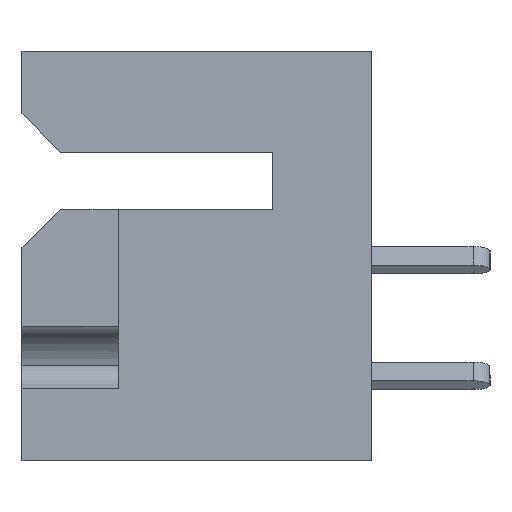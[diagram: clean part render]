
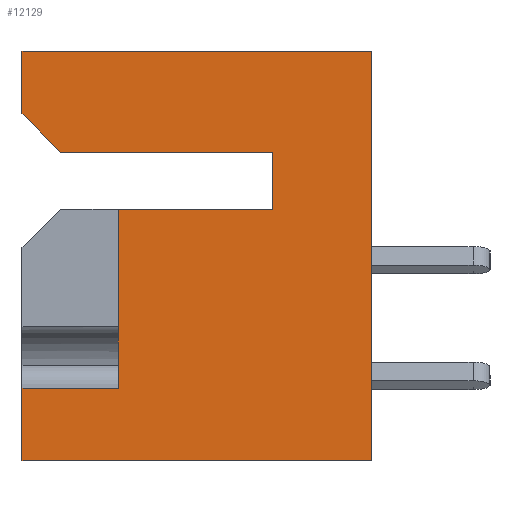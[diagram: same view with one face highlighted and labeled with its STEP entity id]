
A CAD part, left-side view. The second image highlights one B-rep face of the part: STEP entity #12129.
In plain terms, the highlighted planar face has unit normal (-1, 0, 0).
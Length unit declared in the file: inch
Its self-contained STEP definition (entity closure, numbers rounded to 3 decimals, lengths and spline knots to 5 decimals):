
#203 = ORIENTED_EDGE ( 'NONE', *, *, #2435, .F. ) ;
#369 = CARTESIAN_POINT ( 'NONE',  ( 0., 0.328, -0.437 ) ) ;
#496 = DIRECTION ( 'NONE',  ( 0., 1., 0. ) ) ;
#605 = LINE ( 'NONE', #17112, #13194 ) ;
#648 = LINE ( 'NONE', #10663, #18182 ) ;
#671 = DIRECTION ( 'NONE',  ( 0., 1., 0. ) ) ;
#907 = EDGE_CURVE ( 'NONE', #3482, #4054, #5371, .T. ) ;
#1064 = VECTOR ( 'NONE', #8066, 39.37008 ) ;
#1455 = CARTESIAN_POINT ( 'NONE',  ( 0., 0.128, -0.131 ) ) ;
#1504 = CARTESIAN_POINT ( 'NONE',  ( 0., 0.453, -0.081 ) ) ;
#1509 = VERTEX_POINT ( 'NONE', #19637 ) ;
#1584 = VERTEX_POINT ( 'NONE', #2932 ) ;
#1660 = LINE ( 'NONE', #2164, #2198 ) ;
#1769 = CARTESIAN_POINT ( 'NONE',  ( 0., 0.453, 0. ) ) ;
#1850 = DIRECTION ( 'NONE',  ( 0., -0.707, -0.707 ) ) ;
#1857 = LINE ( 'NONE', #14590, #1064 ) ;
#2164 = CARTESIAN_POINT ( 'NONE',  ( 0., 0.328, -0.437 ) ) ;
#2198 = VECTOR ( 'NONE', #496, 39.37008 ) ;
#2222 = EDGE_CURVE ( 'NONE', #15832, #9952, #6212, .T. ) ;
#2435 = EDGE_CURVE ( 'NONE', #15832, #11811, #10362, .T. ) ;
#2499 = DIRECTION ( 'NONE',  ( 0., 0., -1. ) ) ;
#2746 = ORIENTED_EDGE ( 'NONE', *, *, #13058, .F. ) ;
#2792 = VERTEX_POINT ( 'NONE', #369 ) ;
#2932 = CARTESIAN_POINT ( 'NONE',  ( 0., 0., 0. ) ) ;
#3037 = DIRECTION ( 'NONE',  ( 0., 1., 0. ) ) ;
#3432 = VECTOR ( 'NONE', #13560, 39.37008 ) ;
#3482 = VERTEX_POINT ( 'NONE', #6215 ) ;
#3641 = EDGE_CURVE ( 'NONE', #2792, #1509, #1857, .T. ) ;
#3700 = EDGE_CURVE ( 'NONE', #17153, #14867, #10065, .T. ) ;
#4054 = VERTEX_POINT ( 'NONE', #17410 ) ;
#4182 = CARTESIAN_POINT ( 'NONE',  ( 0., 0.453, 0. ) ) ;
#4705 = CARTESIAN_POINT ( 'NONE',  ( 0., 0.453, -0.531 ) ) ;
#5371 = LINE ( 'NONE', #6681, #6901 ) ;
#5588 = ORIENTED_EDGE ( 'NONE', *, *, #3641, .F. ) ;
#5972 = VECTOR ( 'NONE', #19059, 39.37008 ) ;
#6212 = LINE ( 'NONE', #16836, #19392 ) ;
#6215 = CARTESIAN_POINT ( 'NONE',  ( 0., 0.128, -0.205 ) ) ;
#6281 = LINE ( 'NONE', #21240, #12495 ) ;
#6378 = CARTESIAN_POINT ( 'NONE',  ( 0., 0.403, -0.131 ) ) ;
#6535 = DIRECTION ( 'NONE',  ( 0., 0., 1. ) ) ;
#6681 = CARTESIAN_POINT ( 'NONE',  ( 0., 0.128, -0.131 ) ) ;
#6891 = EDGE_CURVE ( 'NONE', #14867, #1584, #648, .T. ) ;
#6901 = VECTOR ( 'NONE', #6535, 39.37008 ) ;
#7118 = CARTESIAN_POINT ( 'NONE',  ( 0., 0., -0.531 ) ) ;
#7164 = LINE ( 'NONE', #1455, #14645 ) ;
#7287 = ORIENTED_EDGE ( 'NONE', *, *, #3700, .T. ) ;
#7370 = EDGE_CURVE ( 'NONE', #2792, #17673, #1660, .T. ) ;
#8011 = EDGE_CURVE ( 'NONE', #17153, #17673, #12193, .T. ) ;
#8066 = DIRECTION ( 'NONE',  ( 0., 0., 1. ) ) ;
#8409 = CARTESIAN_POINT ( 'NONE',  ( 0., 0.453, 0. ) ) ;
#8447 = CARTESIAN_POINT ( 'NONE',  ( 0., 0.453, -0.531 ) ) ;
#9952 = VERTEX_POINT ( 'NONE', #6378 ) ;
#10065 = LINE ( 'NONE', #4705, #13427 ) ;
#10362 = LINE ( 'NONE', #4182, #5972 ) ;
#10663 = CARTESIAN_POINT ( 'NONE',  ( 0., 0., 0. ) ) ;
#10883 = CARTESIAN_POINT ( 'NONE',  ( 0., 0.453, 0. ) ) ;
#11220 = EDGE_CURVE ( 'NONE', #4054, #9952, #7164, .T. ) ;
#11272 = EDGE_LOOP ( 'NONE', ( #16988, #19853, #7287, #20043, #2746, #203, #15900, #20462, #14332, #11787, #5588 ) ) ;
#11350 = DIRECTION ( 'NONE',  ( 0., -1., 0. ) ) ;
#11787 = ORIENTED_EDGE ( 'NONE', *, *, #14834, .T. ) ;
#11811 = VERTEX_POINT ( 'NONE', #1769 ) ;
#12091 = DIRECTION ( 'NONE',  ( 0., 0., 1. ) ) ;
#12129 = ADVANCED_FACE ( 'NONE', ( #17731 ), #20214, .F. ) ;
#12193 = LINE ( 'NONE', #8409, #3432 ) ;
#12495 = VECTOR ( 'NONE', #11350, 39.37008 ) ;
#12849 = CARTESIAN_POINT ( 'NONE',  ( 0., 0.453, -0.437 ) ) ;
#13058 = EDGE_CURVE ( 'NONE', #11811, #1584, #6281, .T. ) ;
#13194 = VECTOR ( 'NONE', #671, 39.37008 ) ;
#13360 = AXIS2_PLACEMENT_3D ( 'NONE', #10883, #19062, #2499 ) ;
#13427 = VECTOR ( 'NONE', #16270, 39.37008 ) ;
#13560 = DIRECTION ( 'NONE',  ( 0., 0., 1. ) ) ;
#14332 = ORIENTED_EDGE ( 'NONE', *, *, #907, .F. ) ;
#14590 = CARTESIAN_POINT ( 'NONE',  ( 0., 0.328, -0.205 ) ) ;
#14645 = VECTOR ( 'NONE', #3037, 39.37008 ) ;
#14834 = EDGE_CURVE ( 'NONE', #3482, #1509, #605, .T. ) ;
#14867 = VERTEX_POINT ( 'NONE', #7118 ) ;
#15832 = VERTEX_POINT ( 'NONE', #1504 ) ;
#15900 = ORIENTED_EDGE ( 'NONE', *, *, #2222, .T. ) ;
#16270 = DIRECTION ( 'NONE',  ( 0., -1., 0. ) ) ;
#16836 = CARTESIAN_POINT ( 'NONE',  ( 0., 0.403, -0.131 ) ) ;
#16988 = ORIENTED_EDGE ( 'NONE', *, *, #7370, .T. ) ;
#17112 = CARTESIAN_POINT ( 'NONE',  ( 0., 0.128, -0.205 ) ) ;
#17153 = VERTEX_POINT ( 'NONE', #8447 ) ;
#17410 = CARTESIAN_POINT ( 'NONE',  ( 0., 0.128, -0.131 ) ) ;
#17673 = VERTEX_POINT ( 'NONE', #12849 ) ;
#17731 = FACE_OUTER_BOUND ( 'NONE', #11272, .T. ) ;
#18182 = VECTOR ( 'NONE', #12091, 39.37008 ) ;
#19059 = DIRECTION ( 'NONE',  ( 0., 0., 1. ) ) ;
#19062 = DIRECTION ( 'NONE',  ( 1., 0., 0. ) ) ;
#19392 = VECTOR ( 'NONE', #1850, 39.37008 ) ;
#19637 = CARTESIAN_POINT ( 'NONE',  ( 0., 0.328, -0.205 ) ) ;
#19853 = ORIENTED_EDGE ( 'NONE', *, *, #8011, .F. ) ;
#20043 = ORIENTED_EDGE ( 'NONE', *, *, #6891, .T. ) ;
#20214 = PLANE ( 'NONE',  #13360 ) ;
#20462 = ORIENTED_EDGE ( 'NONE', *, *, #11220, .F. ) ;
#21240 = CARTESIAN_POINT ( 'NONE',  ( 0., 0.453, 0. ) ) ;
